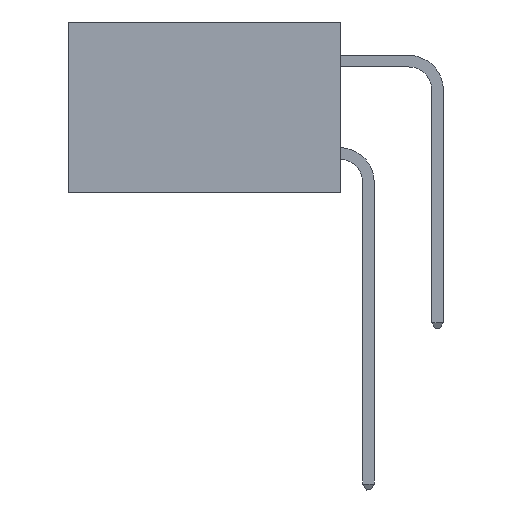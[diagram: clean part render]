
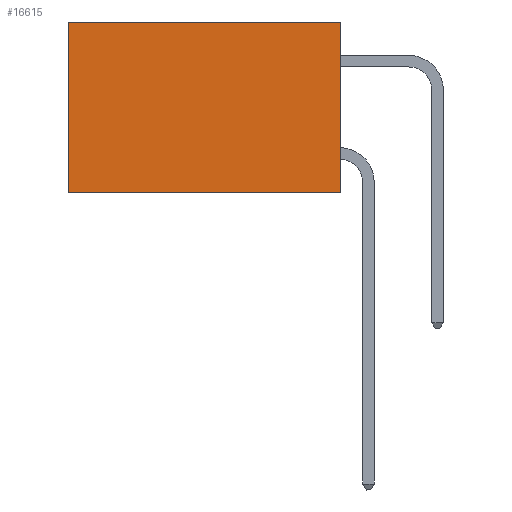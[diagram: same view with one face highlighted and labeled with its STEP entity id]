
A CAD part, left-side view. The second image highlights one B-rep face of the part: STEP entity #16615.
In plain terms, the highlighted planar face has unit normal (-1, 0, 0).
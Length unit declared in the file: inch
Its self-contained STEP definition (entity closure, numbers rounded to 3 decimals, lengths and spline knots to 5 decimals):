
#1083 = CARTESIAN_POINT ( 'NONE',  ( 0.277, 0., -0.37 ) ) ;
#1287 = CARTESIAN_POINT ( 'NONE',  ( 0.277, 0., -0.37 ) ) ;
#1331 = VECTOR ( 'NONE', #13373, 39.37008 ) ;
#1352 = PLANE ( 'NONE',  #11467 ) ;
#2863 = DIRECTION ( 'NONE',  ( 1., 0., 0. ) ) ;
#3207 = VERTEX_POINT ( 'NONE', #11075 ) ;
#3838 = ORIENTED_EDGE ( 'NONE', *, *, #9172, .F. ) ;
#4307 = DIRECTION ( 'NONE',  ( 0., 0., -1. ) ) ;
#4461 = VECTOR ( 'NONE', #13074, 39.37008 ) ;
#4718 = CARTESIAN_POINT ( 'NONE',  ( 0.277, 0., -0.37 ) ) ;
#5627 = VERTEX_POINT ( 'NONE', #4718 ) ;
#5769 = CARTESIAN_POINT ( 'NONE',  ( 0.277, 0.59, 0. ) ) ;
#8453 = LINE ( 'NONE', #1083, #4461 ) ;
#8678 = VECTOR ( 'NONE', #13649, 39.37008 ) ;
#9172 = EDGE_CURVE ( 'NONE', #5627, #14762, #8453, .T. ) ;
#9252 = VERTEX_POINT ( 'NONE', #5769 ) ;
#9434 = EDGE_CURVE ( 'NONE', #3207, #9252, #12206, .T. ) ;
#9495 = ORIENTED_EDGE ( 'NONE', *, *, #11739, .F. ) ;
#10665 = CARTESIAN_POINT ( 'NONE',  ( 0.277, 0., 0. ) ) ;
#11036 = VECTOR ( 'NONE', #4307, 39.37008 ) ;
#11075 = CARTESIAN_POINT ( 'NONE',  ( 0.277, 0., 0. ) ) ;
#11173 = CARTESIAN_POINT ( 'NONE',  ( 0.277, 0.59, -0.37 ) ) ;
#11333 = EDGE_LOOP ( 'NONE', ( #16821, #3838, #9495, #12571 ) ) ;
#11467 = AXIS2_PLACEMENT_3D ( 'NONE', #1287, #2863, #13338 ) ;
#11522 = LINE ( 'NONE', #14750, #11036 ) ;
#11739 = EDGE_CURVE ( 'NONE', #3207, #5627, #13284, .T. ) ;
#11904 = CARTESIAN_POINT ( 'NONE',  ( 0.277, 0., -0.37 ) ) ;
#12206 = LINE ( 'NONE', #10665, #8678 ) ;
#12571 = ORIENTED_EDGE ( 'NONE', *, *, #9434, .T. ) ;
#13074 = DIRECTION ( 'NONE',  ( 0., 1., 0. ) ) ;
#13284 = LINE ( 'NONE', #11904, #1331 ) ;
#13338 = DIRECTION ( 'NONE',  ( 0., 0., -1. ) ) ;
#13373 = DIRECTION ( 'NONE',  ( 0., 0., -1. ) ) ;
#13549 = FACE_OUTER_BOUND ( 'NONE', #11333, .T. ) ;
#13649 = DIRECTION ( 'NONE',  ( 0., 1., 0. ) ) ;
#14750 = CARTESIAN_POINT ( 'NONE',  ( 0.277, 0.59, -0.37 ) ) ;
#14762 = VERTEX_POINT ( 'NONE', #11173 ) ;
#15703 = EDGE_CURVE ( 'NONE', #9252, #14762, #11522, .T. ) ;
#16615 = ADVANCED_FACE ( 'NONE', ( #13549 ), #1352, .F. ) ;
#16821 = ORIENTED_EDGE ( 'NONE', *, *, #15703, .T. ) ;
